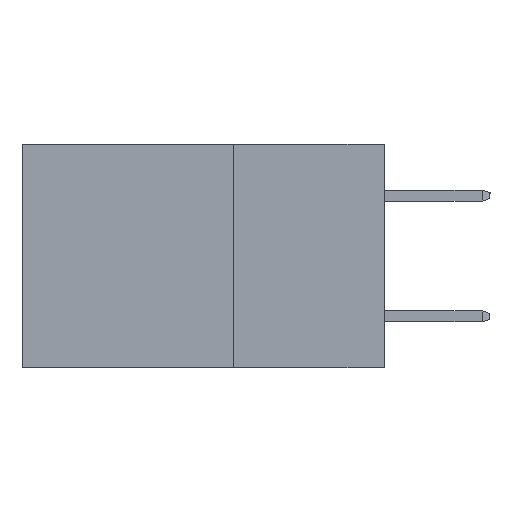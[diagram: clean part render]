
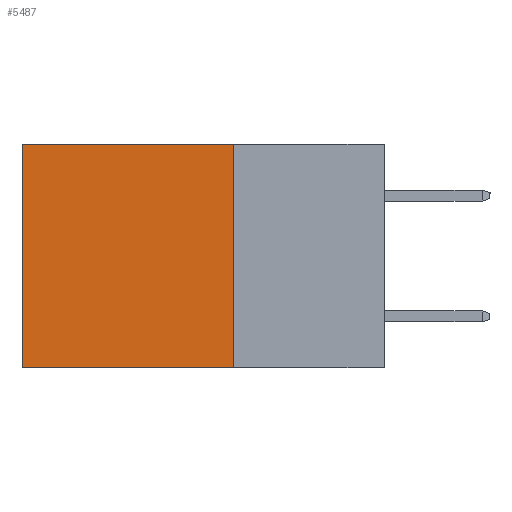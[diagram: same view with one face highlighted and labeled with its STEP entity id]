
A CAD part, left-side view. The second image highlights one B-rep face of the part: STEP entity #5487.
In plain terms, the highlighted planar face has unit normal (-1, 0, 0).
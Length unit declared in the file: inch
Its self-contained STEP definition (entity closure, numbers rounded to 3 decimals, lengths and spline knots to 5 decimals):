
#1203 = ORIENTED_EDGE ( 'NONE', *, *, #23714, .F. ) ;
#1268 = LINE ( 'NONE', #16677, #7294 ) ;
#1869 = FACE_OUTER_BOUND ( 'NONE', #25148, .T. ) ;
#3814 = EDGE_CURVE ( 'NONE', #14172, #18333, #16365, .T. ) ;
#5450 = CARTESIAN_POINT ( 'NONE',  ( 0.2615, 0.6, -0.37 ) ) ;
#5487 = ADVANCED_FACE ( 'NONE', ( #1869 ), #23126, .F. ) ;
#5634 = LINE ( 'NONE', #19826, #9871 ) ;
#5761 = DIRECTION ( 'NONE',  ( 0., 0., -1. ) ) ;
#6078 = DIRECTION ( 'NONE',  ( 0., 1., 0. ) ) ;
#6912 = DIRECTION ( 'NONE',  ( 0., 1., 0. ) ) ;
#7294 = VECTOR ( 'NONE', #6912, 39.37008 ) ;
#7484 = CARTESIAN_POINT ( 'NONE',  ( 0.2615, 0.25, -0.37 ) ) ;
#7971 = ORIENTED_EDGE ( 'NONE', *, *, #12917, .F. ) ;
#8445 = DIRECTION ( 'NONE',  ( 0., 0., -1. ) ) ;
#9871 = VECTOR ( 'NONE', #5761, 39.37008 ) ;
#12030 = ORIENTED_EDGE ( 'NONE', *, *, #17205, .T. ) ;
#12075 = CARTESIAN_POINT ( 'NONE',  ( 0.2615, 0.25, 0. ) ) ;
#12917 = EDGE_CURVE ( 'NONE', #14172, #20807, #23124, .T. ) ;
#13425 = CARTESIAN_POINT ( 'NONE',  ( 0.2615, 0.25, -0.37 ) ) ;
#14172 = VERTEX_POINT ( 'NONE', #23814 ) ;
#15435 = DIRECTION ( 'NONE',  ( 0., 0., -1. ) ) ;
#16365 = LINE ( 'NONE', #12075, #21286 ) ;
#16677 = CARTESIAN_POINT ( 'NONE',  ( 0.2615, 0.25, -0.37 ) ) ;
#17205 = EDGE_CURVE ( 'NONE', #18333, #23822, #5634, .T. ) ;
#17426 = ORIENTED_EDGE ( 'NONE', *, *, #3814, .T. ) ;
#18333 = VERTEX_POINT ( 'NONE', #20149 ) ;
#19328 = CARTESIAN_POINT ( 'NONE',  ( 0.2615, 0.25, -0.37 ) ) ;
#19826 = CARTESIAN_POINT ( 'NONE',  ( 0.2615, 0.6, -0.37 ) ) ;
#20149 = CARTESIAN_POINT ( 'NONE',  ( 0.2615, 0.6, 0. ) ) ;
#20807 = VERTEX_POINT ( 'NONE', #13425 ) ;
#21286 = VECTOR ( 'NONE', #6078, 39.37008 ) ;
#21755 = AXIS2_PLACEMENT_3D ( 'NONE', #7484, #23244, #15435 ) ;
#23124 = LINE ( 'NONE', #19328, #24339 ) ;
#23126 = PLANE ( 'NONE',  #21755 ) ;
#23244 = DIRECTION ( 'NONE',  ( 1., 0., 0. ) ) ;
#23714 = EDGE_CURVE ( 'NONE', #20807, #23822, #1268, .T. ) ;
#23814 = CARTESIAN_POINT ( 'NONE',  ( 0.2615, 0.25, 0. ) ) ;
#23822 = VERTEX_POINT ( 'NONE', #5450 ) ;
#24339 = VECTOR ( 'NONE', #8445, 39.37008 ) ;
#25148 = EDGE_LOOP ( 'NONE', ( #12030, #1203, #7971, #17426 ) ) ;
